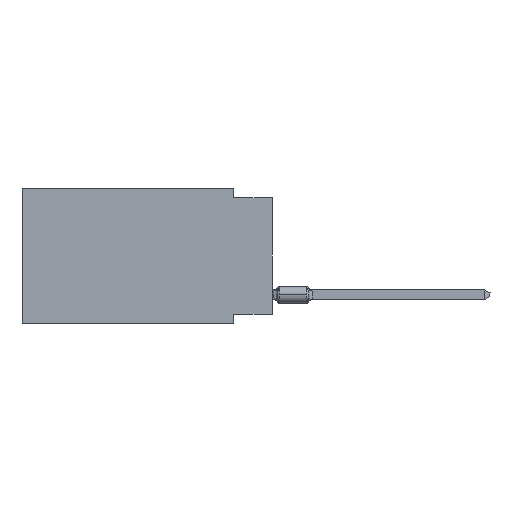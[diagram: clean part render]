
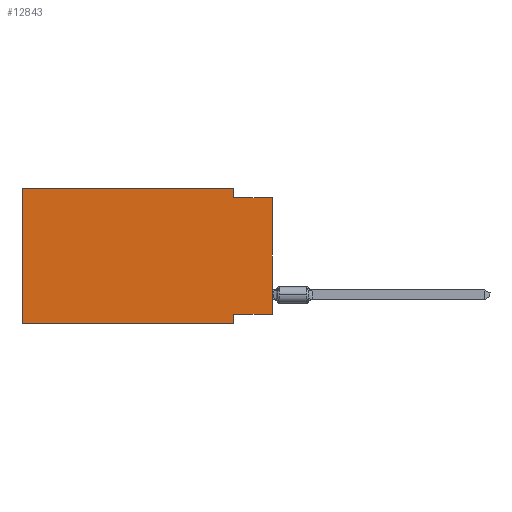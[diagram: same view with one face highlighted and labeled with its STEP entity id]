
A CAD part, left-side view. The second image highlights one B-rep face of the part: STEP entity #12843.
In plain terms, the highlighted planar face has unit normal (-1, 0, 0).
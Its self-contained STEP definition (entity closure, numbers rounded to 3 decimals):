
#6 = ORIENTED_EDGE ( 'NONE', *, *, #27170, .F. ) ;
#1173 = VECTOR ( 'NONE', #8569, 1000. ) ;
#1588 = EDGE_CURVE ( 'NONE', #29465, #20094, #33190, .T. ) ;
#1672 = EDGE_CURVE ( 'NONE', #19268, #32963, #28260, .T. ) ;
#1711 = LINE ( 'NONE', #20485, #8747 ) ;
#2147 = LINE ( 'NONE', #7892, #20783 ) ;
#2696 = VECTOR ( 'NONE', #24392, 1000. ) ;
#3577 = DIRECTION ( 'NONE',  ( 0., 0., 1. ) ) ;
#3849 = ORIENTED_EDGE ( 'NONE', *, *, #9353, .F. ) ;
#4355 = ORIENTED_EDGE ( 'NONE', *, *, #15933, .T. ) ;
#5340 = VERTEX_POINT ( 'NONE', #23488 ) ;
#5571 = CARTESIAN_POINT ( 'NONE',  ( 0., 16.383, -8.89 ) ) ;
#7892 = CARTESIAN_POINT ( 'NONE',  ( 0., 2.54, -8.89 ) ) ;
#8506 = CARTESIAN_POINT ( 'NONE',  ( 0., 16.383, 0. ) ) ;
#8569 = DIRECTION ( 'NONE',  ( 0., 0., -1. ) ) ;
#8644 = EDGE_CURVE ( 'NONE', #32963, #5340, #23962, .T. ) ;
#8747 = VECTOR ( 'NONE', #32515, 1000. ) ;
#9353 = EDGE_CURVE ( 'NONE', #22451, #19268, #1711, .T. ) ;
#9418 = VECTOR ( 'NONE', #18808, 1000. ) ;
#9590 = VERTEX_POINT ( 'NONE', #22911 ) ;
#9620 = EDGE_CURVE ( 'NONE', #20094, #9590, #2147, .T. ) ;
#10008 = DIRECTION ( 'NONE',  ( 1., 0., 0. ) ) ;
#10309 = CARTESIAN_POINT ( 'NONE',  ( 0., 16.383, 0. ) ) ;
#10482 = VECTOR ( 'NONE', #22704, 1000. ) ;
#10614 = EDGE_CURVE ( 'NONE', #29465, #26975, #12477, .T. ) ;
#11245 = DIRECTION ( 'NONE',  ( 0., 0., -1. ) ) ;
#12364 = CARTESIAN_POINT ( 'NONE',  ( 0., 0., -0.635 ) ) ;
#12477 = LINE ( 'NONE', #15654, #24981 ) ;
#12843 = ADVANCED_FACE ( 'NONE', ( #21245 ), #33283, .F. ) ;
#15054 = EDGE_LOOP ( 'NONE', ( #28845, #6, #32191, #22537, #3849, #4355, #17847, #27700 ) ) ;
#15654 = CARTESIAN_POINT ( 'NONE',  ( 0., 0., 0. ) ) ;
#15933 = EDGE_CURVE ( 'NONE', #22451, #9590, #28430, .T. ) ;
#16155 = DIRECTION ( 'NONE',  ( 0., 0., -1. ) ) ;
#17847 = ORIENTED_EDGE ( 'NONE', *, *, #9620, .F. ) ;
#18808 = DIRECTION ( 'NONE',  ( 0., 1., 0. ) ) ;
#19268 = VERTEX_POINT ( 'NONE', #8506 ) ;
#20063 = CARTESIAN_POINT ( 'NONE',  ( 0., 0., -0.635 ) ) ;
#20094 = VERTEX_POINT ( 'NONE', #35879 ) ;
#20124 = VECTOR ( 'NONE', #34199, 1000. ) ;
#20485 = CARTESIAN_POINT ( 'NONE',  ( 0., 16.383, 0. ) ) ;
#20783 = VECTOR ( 'NONE', #11245, 1000. ) ;
#21245 = FACE_OUTER_BOUND ( 'NONE', #15054, .T. ) ;
#22451 = VERTEX_POINT ( 'NONE', #5571 ) ;
#22537 = ORIENTED_EDGE ( 'NONE', *, *, #1672, .F. ) ;
#22704 = DIRECTION ( 'NONE',  ( 0., -1., 0. ) ) ;
#22911 = CARTESIAN_POINT ( 'NONE',  ( 0., 2.54, -8.89 ) ) ;
#23488 = CARTESIAN_POINT ( 'NONE',  ( 0., 2.54, -0.635 ) ) ;
#23962 = LINE ( 'NONE', #35817, #1173 ) ;
#24392 = DIRECTION ( 'NONE',  ( 0., -1., 0. ) ) ;
#24981 = VECTOR ( 'NONE', #3577, 1000. ) ;
#25666 = CARTESIAN_POINT ( 'NONE',  ( 0., 16.383, -8.89 ) ) ;
#26975 = VERTEX_POINT ( 'NONE', #20063 ) ;
#27170 = EDGE_CURVE ( 'NONE', #5340, #26975, #27356, .T. ) ;
#27356 = LINE ( 'NONE', #12364, #2696 ) ;
#27700 = ORIENTED_EDGE ( 'NONE', *, *, #1588, .F. ) ;
#27967 = CARTESIAN_POINT ( 'NONE',  ( 0., 16.383, 0. ) ) ;
#28260 = LINE ( 'NONE', #10309, #20124 ) ;
#28430 = LINE ( 'NONE', #25666, #10482 ) ;
#28845 = ORIENTED_EDGE ( 'NONE', *, *, #10614, .T. ) ;
#29465 = VERTEX_POINT ( 'NONE', #31753 ) ;
#30984 = CARTESIAN_POINT ( 'NONE',  ( 0., 2.54, 0. ) ) ;
#31753 = CARTESIAN_POINT ( 'NONE',  ( 0., 0., -8.255 ) ) ;
#32191 = ORIENTED_EDGE ( 'NONE', *, *, #8644, .F. ) ;
#32515 = DIRECTION ( 'NONE',  ( 0., 0., 1. ) ) ;
#32963 = VERTEX_POINT ( 'NONE', #30984 ) ;
#33190 = LINE ( 'NONE', #33805, #9418 ) ;
#33283 = PLANE ( 'NONE',  #36715 ) ;
#33805 = CARTESIAN_POINT ( 'NONE',  ( 0., 0., -8.255 ) ) ;
#34199 = DIRECTION ( 'NONE',  ( 0., -1., 0. ) ) ;
#35817 = CARTESIAN_POINT ( 'NONE',  ( 0., 2.54, 0. ) ) ;
#35879 = CARTESIAN_POINT ( 'NONE',  ( 0., 2.54, -8.255 ) ) ;
#36715 = AXIS2_PLACEMENT_3D ( 'NONE', #27967, #10008, #16155 ) ;
